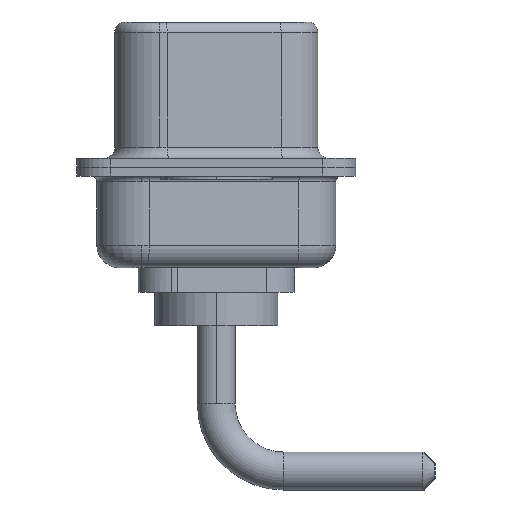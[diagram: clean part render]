
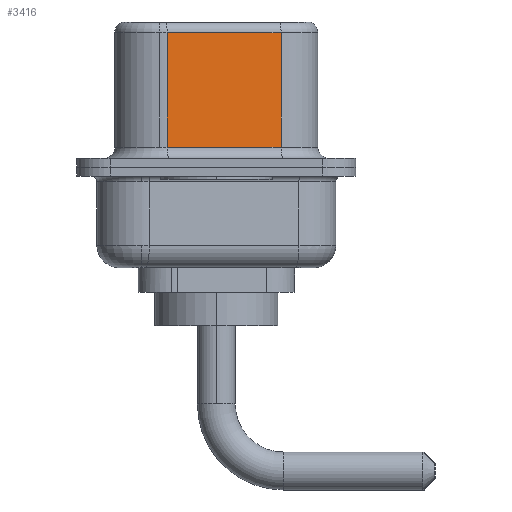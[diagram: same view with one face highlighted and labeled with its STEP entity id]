
A CAD part, left-side view. The second image highlights one B-rep face of the part: STEP entity #3416.
In plain terms, the highlighted planar face has unit normal (-0.985, -0.174, 0).
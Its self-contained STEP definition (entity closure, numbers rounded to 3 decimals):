
#302 = VERTEX_POINT ( 'NONE', #12324 ) ;
#411 = CARTESIAN_POINT ( 'NONE',  ( 4.58, -2.897, 6.02 ) ) ;
#1505 = LINE ( 'NONE', #3662, #7326 ) ;
#1738 = FACE_OUTER_BOUND ( 'NONE', #11946, .T. ) ;
#2570 = LINE ( 'NONE', #5364, #9665 ) ;
#2845 = EDGE_CURVE ( 'NONE', #5997, #6769, #2570, .T. ) ;
#2884 = DIRECTION ( 'NONE',  ( -0.174, 0.985, 0. ) ) ;
#2894 = ORIENTED_EDGE ( 'NONE', *, *, #12502, .T. ) ;
#3416 = ADVANCED_FACE ( 'NONE', ( #1738 ), #8646, .F. ) ;
#3662 = CARTESIAN_POINT ( 'NONE',  ( 3.68, 2.203, 6.52 ) ) ;
#4604 = CARTESIAN_POINT ( 'NONE',  ( 4.58, -2.897, 6.02 ) ) ;
#4621 = AXIS2_PLACEMENT_3D ( 'NONE', #11311, #10482, #4772 ) ;
#4772 = DIRECTION ( 'NONE',  ( -0.174, 0.985, 0. ) ) ;
#5364 = CARTESIAN_POINT ( 'NONE',  ( 4.58, -2.897, 6.52 ) ) ;
#5997 = VERTEX_POINT ( 'NONE', #411 ) ;
#6769 = VERTEX_POINT ( 'NONE', #9857 ) ;
#7224 = ORIENTED_EDGE ( 'NONE', *, *, #2845, .F. ) ;
#7326 = VECTOR ( 'NONE', #10447, 1000. ) ;
#7369 = CARTESIAN_POINT ( 'NONE',  ( 4.58, -2.897, 0.9 ) ) ;
#7467 = EDGE_CURVE ( 'NONE', #11652, #6769, #12318, .T. ) ;
#7876 = ORIENTED_EDGE ( 'NONE', *, *, #7467, .T. ) ;
#8324 = ORIENTED_EDGE ( 'NONE', *, *, #9564, .T. ) ;
#8646 = PLANE ( 'NONE',  #4621 ) ;
#9110 = VECTOR ( 'NONE', #2884, 1000. ) ;
#9241 = DIRECTION ( 'NONE',  ( 0., 0., -1. ) ) ;
#9564 = EDGE_CURVE ( 'NONE', #5997, #302, #12420, .T. ) ;
#9586 = VECTOR ( 'NONE', #11234, 1000. ) ;
#9665 = VECTOR ( 'NONE', #9241, 1000. ) ;
#9857 = CARTESIAN_POINT ( 'NONE',  ( 4.58, -2.897, 0.9 ) ) ;
#10447 = DIRECTION ( 'NONE',  ( 0., 0., -1. ) ) ;
#10482 = DIRECTION ( 'NONE',  ( 0.985, 0.174, 0. ) ) ;
#11234 = DIRECTION ( 'NONE',  ( 0.174, -0.985, 0. ) ) ;
#11311 = CARTESIAN_POINT ( 'NONE',  ( 4.58, -2.897, 6.52 ) ) ;
#11652 = VERTEX_POINT ( 'NONE', #12569 ) ;
#11946 = EDGE_LOOP ( 'NONE', ( #7224, #8324, #2894, #7876 ) ) ;
#12318 = LINE ( 'NONE', #7369, #9586 ) ;
#12324 = CARTESIAN_POINT ( 'NONE',  ( 3.68, 2.203, 6.02 ) ) ;
#12420 = LINE ( 'NONE', #4604, #9110 ) ;
#12502 = EDGE_CURVE ( 'NONE', #302, #11652, #1505, .T. ) ;
#12569 = CARTESIAN_POINT ( 'NONE',  ( 3.68, 2.203, 0.9 ) ) ;
